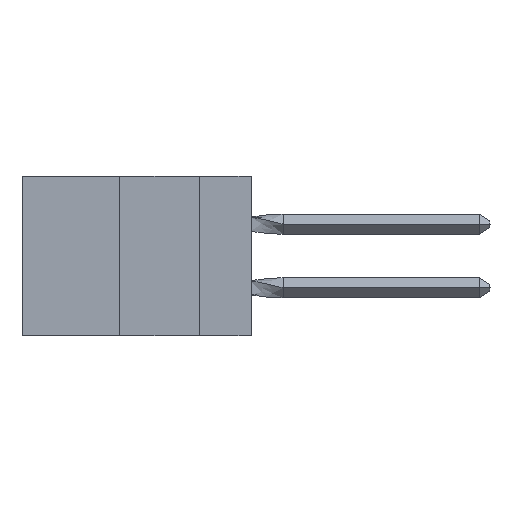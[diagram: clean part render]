
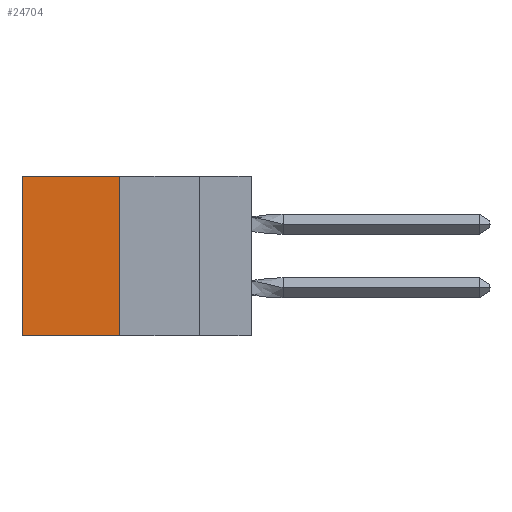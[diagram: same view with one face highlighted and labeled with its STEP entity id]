
A CAD part, left-side view. The second image highlights one B-rep face of the part: STEP entity #24704.
In plain terms, the highlighted planar face has unit normal (-1, 0, 0).
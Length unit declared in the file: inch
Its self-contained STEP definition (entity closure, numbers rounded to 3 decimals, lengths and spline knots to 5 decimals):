
#105 = EDGE_CURVE ( 'NONE', #13610, #12339, #30893, .T. ) ;
#2213 = EDGE_CURVE ( 'NONE', #13610, #19790, #17143, .T. ) ;
#4484 = DIRECTION ( 'NONE',  ( 0., 0., -1. ) ) ;
#4499 = VECTOR ( 'NONE', #4484, 39.37008 ) ;
#6358 = CARTESIAN_POINT ( 'NONE',  ( 0.305, 0.413, -0.5 ) ) ;
#7785 = VECTOR ( 'NONE', #25003, 39.37008 ) ;
#8328 = DIRECTION ( 'NONE',  ( 0., 1., 0. ) ) ;
#8974 = CARTESIAN_POINT ( 'NONE',  ( 0.305, 0.413, 0. ) ) ;
#9192 = CARTESIAN_POINT ( 'NONE',  ( 0.305, 0.72, -0.5 ) ) ;
#10791 = EDGE_CURVE ( 'NONE', #12339, #20157, #28644, .T. ) ;
#10994 = VECTOR ( 'NONE', #31196, 39.37008 ) ;
#11196 = CARTESIAN_POINT ( 'NONE',  ( 0.305, 0.72, -0.5 ) ) ;
#11497 = DIRECTION ( 'NONE',  ( 1., 0., 0. ) ) ;
#11908 = LINE ( 'NONE', #19635, #13494 ) ;
#12339 = VERTEX_POINT ( 'NONE', #19628 ) ;
#13026 = CARTESIAN_POINT ( 'NONE',  ( 0.305, 0.413, -0.5 ) ) ;
#13229 = CARTESIAN_POINT ( 'NONE',  ( 0.305, 0.413, 0. ) ) ;
#13494 = VECTOR ( 'NONE', #8328, 39.37008 ) ;
#13610 = VERTEX_POINT ( 'NONE', #13229 ) ;
#16887 = ORIENTED_EDGE ( 'NONE', *, *, #10791, .T. ) ;
#17143 = LINE ( 'NONE', #13026, #7785 ) ;
#19342 = FACE_OUTER_BOUND ( 'NONE', #22115, .T. ) ;
#19628 = CARTESIAN_POINT ( 'NONE',  ( 0.305, 0.72, 0. ) ) ;
#19635 = CARTESIAN_POINT ( 'NONE',  ( 0.305, 0.413, -0.5 ) ) ;
#19790 = VERTEX_POINT ( 'NONE', #6358 ) ;
#20157 = VERTEX_POINT ( 'NONE', #11196 ) ;
#21299 = PLANE ( 'NONE',  #24203 ) ;
#22115 = EDGE_LOOP ( 'NONE', ( #16887, #29023, #27408, #25116 ) ) ;
#24203 = AXIS2_PLACEMENT_3D ( 'NONE', #26414, #11497, #28910 ) ;
#24704 = ADVANCED_FACE ( 'NONE', ( #19342 ), #21299, .F. ) ;
#25003 = DIRECTION ( 'NONE',  ( 0., 0., -1. ) ) ;
#25005 = EDGE_CURVE ( 'NONE', #19790, #20157, #11908, .T. ) ;
#25116 = ORIENTED_EDGE ( 'NONE', *, *, #105, .T. ) ;
#26414 = CARTESIAN_POINT ( 'NONE',  ( 0.305, 0.413, -0.5 ) ) ;
#27408 = ORIENTED_EDGE ( 'NONE', *, *, #2213, .F. ) ;
#28644 = LINE ( 'NONE', #9192, #4499 ) ;
#28910 = DIRECTION ( 'NONE',  ( 0., 0., -1. ) ) ;
#29023 = ORIENTED_EDGE ( 'NONE', *, *, #25005, .F. ) ;
#30893 = LINE ( 'NONE', #8974, #10994 ) ;
#31196 = DIRECTION ( 'NONE',  ( 0., 1., 0. ) ) ;
